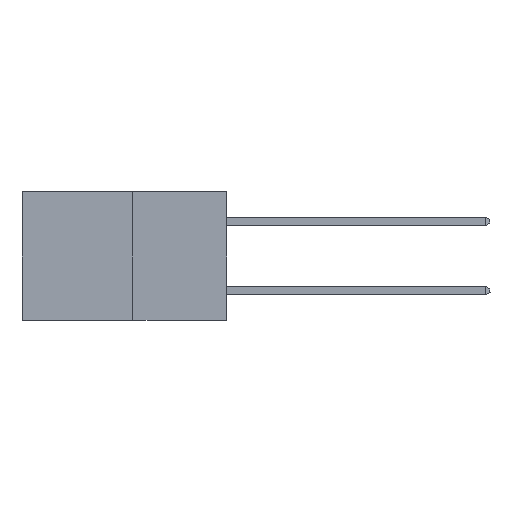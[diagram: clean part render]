
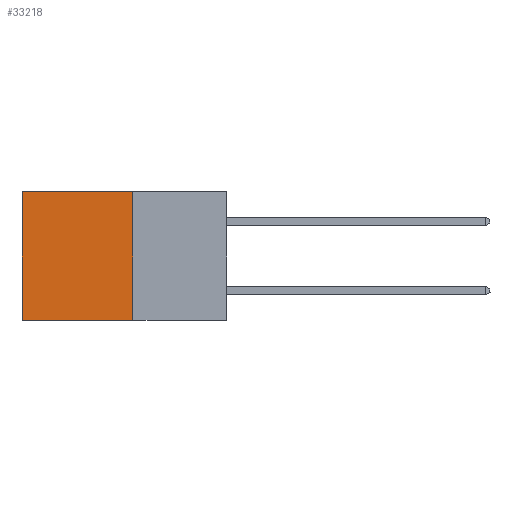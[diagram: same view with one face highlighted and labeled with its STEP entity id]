
A CAD part, left-side view. The second image highlights one B-rep face of the part: STEP entity #33218.
In plain terms, the highlighted planar face has unit normal (-1, 0, 0).
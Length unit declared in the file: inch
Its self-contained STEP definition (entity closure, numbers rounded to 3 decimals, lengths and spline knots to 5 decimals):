
#2272 = CARTESIAN_POINT ( 'NONE',  ( 0.277, 0.27, 0. ) ) ;
#2696 = VECTOR ( 'NONE', #11690, 39.37008 ) ;
#4295 = EDGE_CURVE ( 'NONE', #7306, #30850, #13751, .T. ) ;
#5461 = FACE_OUTER_BOUND ( 'NONE', #9802, .T. ) ;
#6754 = ORIENTED_EDGE ( 'NONE', *, *, #9613, .T. ) ;
#7306 = VERTEX_POINT ( 'NONE', #25985 ) ;
#9392 = AXIS2_PLACEMENT_3D ( 'NONE', #31974, #15727, #34703 ) ;
#9613 = EDGE_CURVE ( 'NONE', #13593, #7306, #17302, .T. ) ;
#9802 = EDGE_LOOP ( 'NONE', ( #19326, #20195, #33326, #6754 ) ) ;
#11440 = LINE ( 'NONE', #13922, #30603 ) ;
#11469 = CARTESIAN_POINT ( 'NONE',  ( 0.277, 0.59, -0.37 ) ) ;
#11690 = DIRECTION ( 'NONE',  ( 0., 1., 0. ) ) ;
#13593 = VERTEX_POINT ( 'NONE', #2272 ) ;
#13751 = LINE ( 'NONE', #11469, #27414 ) ;
#13922 = CARTESIAN_POINT ( 'NONE',  ( 0.277, 0.27, -0.37 ) ) ;
#14598 = DIRECTION ( 'NONE',  ( 0., 0., -1. ) ) ;
#14684 = VECTOR ( 'NONE', #14598, 39.37008 ) ;
#15727 = DIRECTION ( 'NONE',  ( 1., 0., 0. ) ) ;
#17176 = VERTEX_POINT ( 'NONE', #17601 ) ;
#17302 = LINE ( 'NONE', #25297, #2696 ) ;
#17601 = CARTESIAN_POINT ( 'NONE',  ( 0.277, 0.27, -0.37 ) ) ;
#19326 = ORIENTED_EDGE ( 'NONE', *, *, #4295, .T. ) ;
#19669 = CARTESIAN_POINT ( 'NONE',  ( 0.277, 0.59, -0.37 ) ) ;
#20195 = ORIENTED_EDGE ( 'NONE', *, *, #33485, .F. ) ;
#21096 = PLANE ( 'NONE',  #9392 ) ;
#22160 = DIRECTION ( 'NONE',  ( 0., 1., 0. ) ) ;
#22741 = CARTESIAN_POINT ( 'NONE',  ( 0.277, 0.27, -0.37 ) ) ;
#25297 = CARTESIAN_POINT ( 'NONE',  ( 0.277, 0.27, 0. ) ) ;
#25985 = CARTESIAN_POINT ( 'NONE',  ( 0.277, 0.59, 0. ) ) ;
#27414 = VECTOR ( 'NONE', #33197, 39.37008 ) ;
#29343 = EDGE_CURVE ( 'NONE', #13593, #17176, #30849, .T. ) ;
#30603 = VECTOR ( 'NONE', #22160, 39.37008 ) ;
#30850 = VERTEX_POINT ( 'NONE', #19669 ) ;
#30849 = LINE ( 'NONE', #22741, #14684 ) ;
#31974 = CARTESIAN_POINT ( 'NONE',  ( 0.277, 0.27, -0.37 ) ) ;
#33197 = DIRECTION ( 'NONE',  ( 0., 0., -1. ) ) ;
#33218 = ADVANCED_FACE ( 'NONE', ( #5461 ), #21096, .F. ) ;
#33326 = ORIENTED_EDGE ( 'NONE', *, *, #29343, .F. ) ;
#33485 = EDGE_CURVE ( 'NONE', #17176, #30850, #11440, .T. ) ;
#34703 = DIRECTION ( 'NONE',  ( 0., 0., -1. ) ) ;
